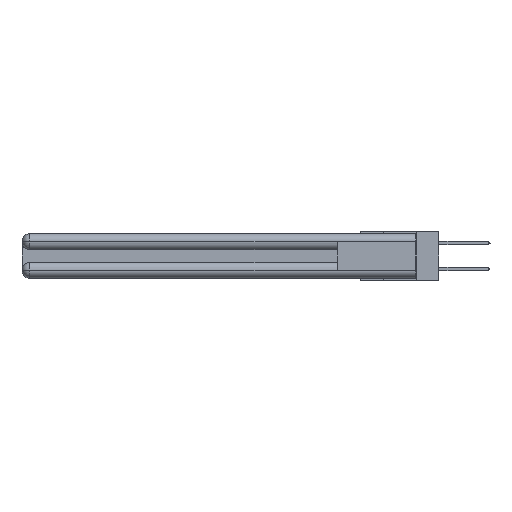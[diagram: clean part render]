
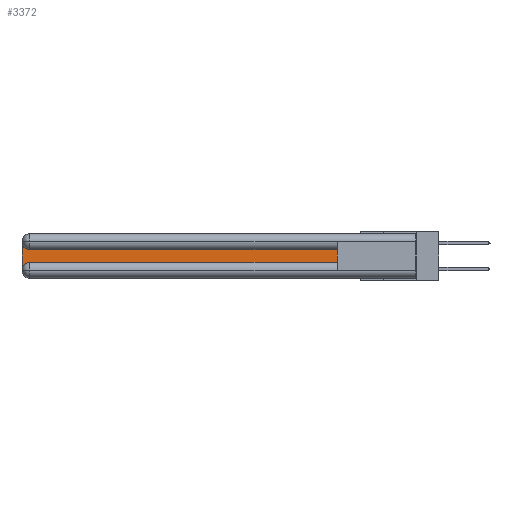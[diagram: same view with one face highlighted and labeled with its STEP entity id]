
A CAD part, left-side view. The second image highlights one B-rep face of the part: STEP entity #3372.
In plain terms, the highlighted planar face has unit normal (-1, 0, 0).
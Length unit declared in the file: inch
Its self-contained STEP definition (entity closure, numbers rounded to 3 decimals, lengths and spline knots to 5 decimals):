
#328 = DIRECTION ( 'NONE',  ( 0., 0., -1. ) ) ;
#1248 = DIRECTION ( 'NONE',  ( 0., 0., -1. ) ) ;
#2616 = CIRCLE ( 'NONE', #5384, 0.06 ) ;
#3372 = ADVANCED_FACE ( 'NONE', ( #11273 ), #13589, .F. ) ;
#3416 = ORIENTED_EDGE ( 'NONE', *, *, #17091, .T. ) ;
#3956 = LINE ( 'NONE', #16569, #6290 ) ;
#4282 = ORIENTED_EDGE ( 'NONE', *, *, #27984, .T. ) ;
#4381 = VECTOR ( 'NONE', #20374, 39.37008 ) ;
#4888 = CARTESIAN_POINT ( 'NONE',  ( 0.075, 3., -0.0625 ) ) ;
#5384 = AXIS2_PLACEMENT_3D ( 'NONE', #20722, #5661, #13027 ) ;
#5661 = DIRECTION ( 'NONE',  ( 1., 0., 0. ) ) ;
#5891 = CARTESIAN_POINT ( 'NONE',  ( 0.075, 3., -0.1225 ) ) ;
#6290 = VECTOR ( 'NONE', #22087, 39.37008 ) ;
#6853 = AXIS2_PLACEMENT_3D ( 'NONE', #11541, #16124, #1248 ) ;
#8602 = AXIS2_PLACEMENT_3D ( 'NONE', #5891, #28350, #328 ) ;
#8975 = VECTOR ( 'NONE', #30828, 39.37008 ) ;
#9161 = EDGE_CURVE ( 'NONE', #13468, #29104, #3956, .T. ) ;
#10925 = CARTESIAN_POINT ( 'NONE',  ( 0.075, 0.6, -0.2175 ) ) ;
#11273 = FACE_OUTER_BOUND ( 'NONE', #24634, .T. ) ;
#11522 = ORIENTED_EDGE ( 'NONE', *, *, #9161, .T. ) ;
#11541 = CARTESIAN_POINT ( 'NONE',  ( 0.075, 2.94, -0.0625 ) ) ;
#12757 = CARTESIAN_POINT ( 'NONE',  ( 0.075, 0.6, -0.2175 ) ) ;
#12998 = ORIENTED_EDGE ( 'NONE', *, *, #20959, .T. ) ;
#13027 = DIRECTION ( 'NONE',  ( 0., 0., -1. ) ) ;
#13468 = VERTEX_POINT ( 'NONE', #4888 ) ;
#13521 = VERTEX_POINT ( 'NONE', #19762 ) ;
#13589 = PLANE ( 'NONE',  #8602 ) ;
#14243 = CIRCLE ( 'NONE', #6853, 0.06 ) ;
#16124 = DIRECTION ( 'NONE',  ( 1., 0., 0. ) ) ;
#16569 = CARTESIAN_POINT ( 'NONE',  ( 0.075, 3., -0.2175 ) ) ;
#16709 = LINE ( 'NONE', #30609, #8975 ) ;
#17091 = EDGE_CURVE ( 'NONE', #23975, #22857, #16709, .T. ) ;
#18041 = ORIENTED_EDGE ( 'NONE', *, *, #25378, .T. ) ;
#19762 = CARTESIAN_POINT ( 'NONE',  ( 0.075, 2.94, -0.2175 ) ) ;
#20374 = DIRECTION ( 'NONE',  ( 0., 1., 0. ) ) ;
#20722 = CARTESIAN_POINT ( 'NONE',  ( 0.075, 2.94, -0.2775 ) ) ;
#20959 = EDGE_CURVE ( 'NONE', #22857, #28252, #31514, .T. ) ;
#21632 = CARTESIAN_POINT ( 'NONE',  ( 0.075, 2.94, -0.1225 ) ) ;
#21801 = VECTOR ( 'NONE', #28179, 39.37008 ) ;
#22087 = DIRECTION ( 'NONE',  ( 0., 0., -1. ) ) ;
#22857 = VERTEX_POINT ( 'NONE', #30905 ) ;
#23300 = CARTESIAN_POINT ( 'NONE',  ( 0.075, 3., -0.2775 ) ) ;
#23408 = EDGE_CURVE ( 'NONE', #29104, #13521, #2616, .T. ) ;
#23975 = VERTEX_POINT ( 'NONE', #12757 ) ;
#24127 = LINE ( 'NONE', #10925, #21801 ) ;
#24634 = EDGE_LOOP ( 'NONE', ( #12998, #18041, #11522, #29881, #4282, #3416 ) ) ;
#25343 = CARTESIAN_POINT ( 'NONE',  ( 0.075, 0.6, -0.1225 ) ) ;
#25378 = EDGE_CURVE ( 'NONE', #28252, #13468, #14243, .T. ) ;
#27984 = EDGE_CURVE ( 'NONE', #13521, #23975, #24127, .T. ) ;
#28179 = DIRECTION ( 'NONE',  ( 0., -1., 0. ) ) ;
#28252 = VERTEX_POINT ( 'NONE', #21632 ) ;
#28350 = DIRECTION ( 'NONE',  ( 1., 0., 0. ) ) ;
#29104 = VERTEX_POINT ( 'NONE', #23300 ) ;
#29881 = ORIENTED_EDGE ( 'NONE', *, *, #23408, .T. ) ;
#30609 = CARTESIAN_POINT ( 'NONE',  ( 0.075, 0.6, -0.2175 ) ) ;
#30828 = DIRECTION ( 'NONE',  ( 0., 0., 1. ) ) ;
#30905 = CARTESIAN_POINT ( 'NONE',  ( 0.075, 0.6, -0.1225 ) ) ;
#31514 = LINE ( 'NONE', #25343, #4381 ) ;
